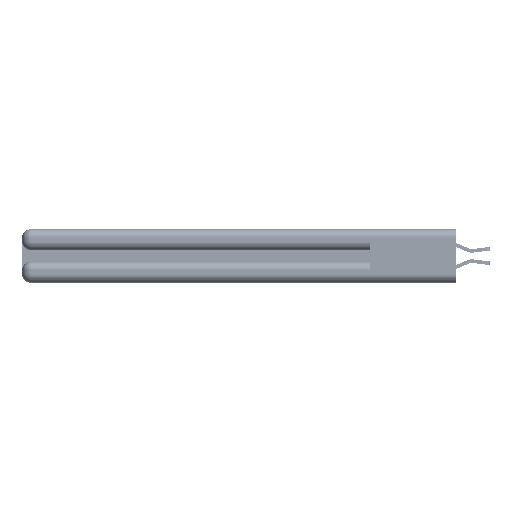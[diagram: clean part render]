
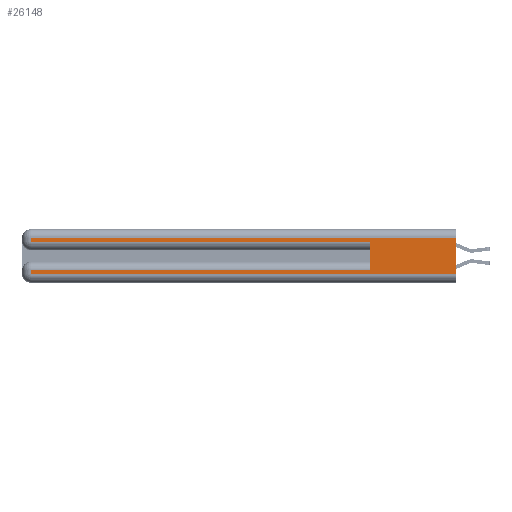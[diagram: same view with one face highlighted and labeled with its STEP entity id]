
A CAD part, left-side view. The second image highlights one B-rep face of the part: STEP entity #26148.
In plain terms, the highlighted planar face has unit normal (-1, 0, 0).
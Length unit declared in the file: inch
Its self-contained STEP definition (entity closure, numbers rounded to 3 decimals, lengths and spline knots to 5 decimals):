
#317 = CARTESIAN_POINT ( 'NONE',  ( 0., 0., 0.085 ) ) ;
#954 = CARTESIAN_POINT ( 'NONE',  ( 0., 0., 0.06 ) ) ;
#1077 = EDGE_CURVE ( 'NONE', #41300, #4480, #2326, .T. ) ;
#2326 = LINE ( 'NONE', #30323, #48129 ) ;
#4480 = VERTEX_POINT ( 'NONE', #16008 ) ;
#6665 = EDGE_CURVE ( 'NONE', #43290, #4480, #49820, .T. ) ;
#8100 = VECTOR ( 'NONE', #27877, 39.37008 ) ;
#8203 = ORIENTED_EDGE ( 'NONE', *, *, #6665, .F. ) ;
#9622 = ORIENTED_EDGE ( 'NONE', *, *, #12997, .T. ) ;
#9963 = LINE ( 'NONE', #44386, #33627 ) ;
#10649 = CARTESIAN_POINT ( 'NONE',  ( 0., 0., 0.37 ) ) ;
#12997 = EDGE_CURVE ( 'NONE', #43290, #24190, #27924, .T. ) ;
#13377 = VERTEX_POINT ( 'NONE', #55871 ) ;
#14551 = VECTOR ( 'NONE', #46953, 39.37008 ) ;
#15110 = DIRECTION ( 'NONE',  ( 0., 0., -1. ) ) ;
#16008 = CARTESIAN_POINT ( 'NONE',  ( 0., 0.6, 0.285 ) ) ;
#16563 = CARTESIAN_POINT ( 'NONE',  ( 0., 2.94, 0.085 ) ) ;
#17327 = ORIENTED_EDGE ( 'NONE', *, *, #18193, .T. ) ;
#17874 = DIRECTION ( 'NONE',  ( 0., 0., -1. ) ) ;
#18193 = EDGE_CURVE ( 'NONE', #30065, #13377, #19962, .T. ) ;
#19962 = LINE ( 'NONE', #954, #8100 ) ;
#20942 = EDGE_CURVE ( 'NONE', #55481, #41300, #45313, .T. ) ;
#21051 = LINE ( 'NONE', #56520, #53423 ) ;
#21594 = DIRECTION ( 'NONE',  ( 0., -1., 0. ) ) ;
#21677 = CARTESIAN_POINT ( 'NONE',  ( 0., 0.6, 0.085 ) ) ;
#21731 = EDGE_CURVE ( 'NONE', #46703, #13377, #21051, .T. ) ;
#22645 = DIRECTION ( 'NONE',  ( 0., 1., 0. ) ) ;
#23587 = DIRECTION ( 'NONE',  ( 0., 0., -1. ) ) ;
#24190 = VERTEX_POINT ( 'NONE', #16563 ) ;
#26148 = ADVANCED_FACE ( 'NONE', ( #37238 ), #32811, .F. ) ;
#26551 = VECTOR ( 'NONE', #22645, 39.37008 ) ;
#27341 = AXIS2_PLACEMENT_3D ( 'NONE', #10649, #41621, #15110 ) ;
#27877 = DIRECTION ( 'NONE',  ( 0., -1., 0. ) ) ;
#27924 = LINE ( 'NONE', #317, #26551 ) ;
#29900 = VECTOR ( 'NONE', #31973, 39.37008 ) ;
#30065 = VERTEX_POINT ( 'NONE', #55079 ) ;
#30224 = DIRECTION ( 'NONE',  ( 0., 0., -1. ) ) ;
#30323 = CARTESIAN_POINT ( 'NONE',  ( 0., 0., 0.285 ) ) ;
#31973 = DIRECTION ( 'NONE',  ( 0., 1., 0. ) ) ;
#32289 = CARTESIAN_POINT ( 'NONE',  ( 0., 2.94, 0.37 ) ) ;
#32811 = PLANE ( 'NONE',  #27341 ) ;
#33627 = VECTOR ( 'NONE', #17874, 39.37008 ) ;
#33644 = VECTOR ( 'NONE', #23587, 39.37008 ) ;
#35987 = EDGE_LOOP ( 'NONE', ( #47677, #38729, #41460, #36677, #8203, #9622, #47064, #17327 ) ) ;
#36677 = ORIENTED_EDGE ( 'NONE', *, *, #1077, .T. ) ;
#37238 = FACE_OUTER_BOUND ( 'NONE', #35987, .T. ) ;
#38729 = ORIENTED_EDGE ( 'NONE', *, *, #55273, .T. ) ;
#41300 = VERTEX_POINT ( 'NONE', #54366 ) ;
#41460 = ORIENTED_EDGE ( 'NONE', *, *, #20942, .T. ) ;
#41587 = LINE ( 'NONE', #54006, #29900 ) ;
#41621 = DIRECTION ( 'NONE',  ( 1., 0., 0. ) ) ;
#41908 = EDGE_CURVE ( 'NONE', #24190, #30065, #9963, .T. ) ;
#42527 = CARTESIAN_POINT ( 'NONE',  ( 0., 0.6, 0.145 ) ) ;
#42917 = CARTESIAN_POINT ( 'NONE',  ( 0., 0., 0.31 ) ) ;
#43290 = VERTEX_POINT ( 'NONE', #21677 ) ;
#44386 = CARTESIAN_POINT ( 'NONE',  ( 0., 2.94, 0.37 ) ) ;
#45313 = LINE ( 'NONE', #32289, #33644 ) ;
#46703 = VERTEX_POINT ( 'NONE', #42917 ) ;
#46953 = DIRECTION ( 'NONE',  ( 0., 0., 1. ) ) ;
#47064 = ORIENTED_EDGE ( 'NONE', *, *, #41908, .T. ) ;
#47677 = ORIENTED_EDGE ( 'NONE', *, *, #21731, .F. ) ;
#48129 = VECTOR ( 'NONE', #21594, 39.37008 ) ;
#49820 = LINE ( 'NONE', #42527, #14551 ) ;
#50932 = CARTESIAN_POINT ( 'NONE',  ( 0., 2.94, 0.31 ) ) ;
#53423 = VECTOR ( 'NONE', #30224, 39.37008 ) ;
#54006 = CARTESIAN_POINT ( 'NONE',  ( 0., 0., 0.31 ) ) ;
#54366 = CARTESIAN_POINT ( 'NONE',  ( 0., 2.94, 0.285 ) ) ;
#55079 = CARTESIAN_POINT ( 'NONE',  ( 0., 2.94, 0.06 ) ) ;
#55273 = EDGE_CURVE ( 'NONE', #46703, #55481, #41587, .T. ) ;
#55481 = VERTEX_POINT ( 'NONE', #50932 ) ;
#55871 = CARTESIAN_POINT ( 'NONE',  ( 0., 0., 0.06 ) ) ;
#56520 = CARTESIAN_POINT ( 'NONE',  ( 0., 0., 0.37 ) ) ;
